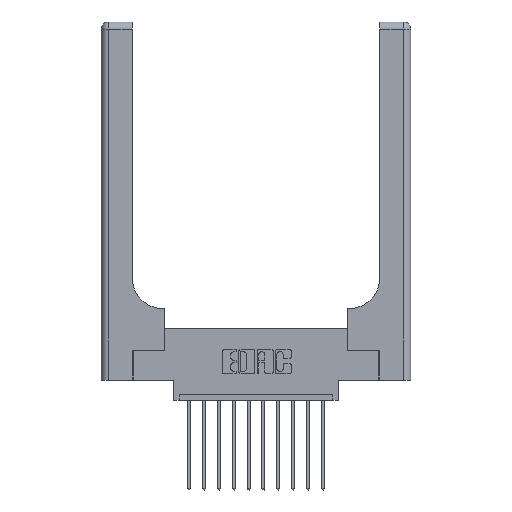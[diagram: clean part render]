
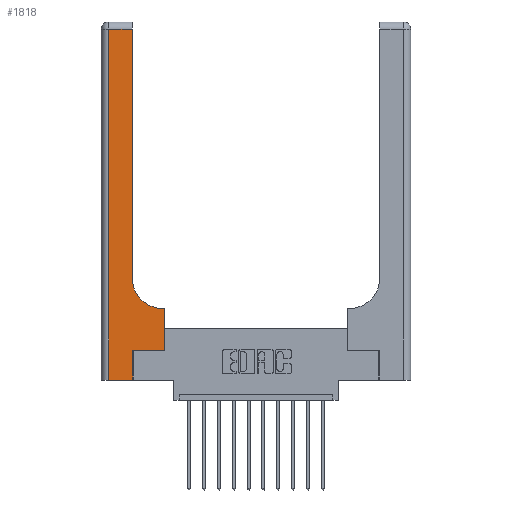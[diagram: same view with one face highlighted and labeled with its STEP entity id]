
A CAD part, top view. The second image highlights one B-rep face of the part: STEP entity #1818.
In plain terms, the highlighted planar face has unit normal (0, 0, 1).
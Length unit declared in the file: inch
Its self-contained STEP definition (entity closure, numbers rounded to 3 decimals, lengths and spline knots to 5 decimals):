
#231 = EDGE_CURVE ( 'NONE', #11655, #13411, #13240, .T. ) ;
#300 = DIRECTION ( 'NONE',  ( 1., 0., 0. ) ) ;
#375 = LINE ( 'NONE', #10136, #12994 ) ;
#502 = LINE ( 'NONE', #2709, #3537 ) ;
#524 = EDGE_LOOP ( 'NONE', ( #6672, #3732, #3920, #12503, #13921, #8784, #4140, #12211, #5558 ) ) ;
#971 = CARTESIAN_POINT ( 'NONE',  ( 0.06, 2.94, 0.37 ) ) ;
#1190 = LINE ( 'NONE', #6204, #11714 ) ;
#1419 = EDGE_CURVE ( 'NONE', #5916, #8251, #5658, .T. ) ;
#1541 = DIRECTION ( 'NONE',  ( 1., 0., 0. ) ) ;
#1778 = VECTOR ( 'NONE', #8860, 39.37008 ) ;
#1818 = ADVANCED_FACE ( 'NONE', ( #9662 ), #10863, .F. ) ;
#2227 = CARTESIAN_POINT ( 'NONE',  ( 0.51, 0.6, 0.37 ) ) ;
#2591 = CARTESIAN_POINT ( 'NONE',  ( 0.265, 0., 0.37 ) ) ;
#2709 = CARTESIAN_POINT ( 'NONE',  ( 0.26, 0.6, 0.37 ) ) ;
#3477 = EDGE_CURVE ( 'NONE', #13411, #10782, #11350, .T. ) ;
#3537 = VECTOR ( 'NONE', #4005, 39.37008 ) ;
#3730 = CARTESIAN_POINT ( 'NONE',  ( 0.528, 0.25, 0.37 ) ) ;
#3732 = ORIENTED_EDGE ( 'NONE', *, *, #231, .T. ) ;
#3757 = CARTESIAN_POINT ( 'NONE',  ( 0., 0., 0.37 ) ) ;
#3920 = ORIENTED_EDGE ( 'NONE', *, *, #3477, .T. ) ;
#4005 = DIRECTION ( 'NONE',  ( -1., 0., 0. ) ) ;
#4070 = EDGE_CURVE ( 'NONE', #8092, #7566, #1190, .T. ) ;
#4140 = ORIENTED_EDGE ( 'NONE', *, *, #1419, .T. ) ;
#4496 = EDGE_CURVE ( 'NONE', #8410, #8673, #9220, .T. ) ;
#4697 = CARTESIAN_POINT ( 'NONE',  ( 0., 3., 0.37 ) ) ;
#4716 = DIRECTION ( 'NONE',  ( 0., -1., 0. ) ) ;
#5558 = ORIENTED_EDGE ( 'NONE', *, *, #4496, .T. ) ;
#5658 = LINE ( 'NONE', #3730, #12937 ) ;
#5916 = VERTEX_POINT ( 'NONE', #9123 ) ;
#5938 = DIRECTION ( 'NONE',  ( 0., 0., -1. ) ) ;
#6204 = CARTESIAN_POINT ( 'NONE',  ( 0.265, 0., 0.37 ) ) ;
#6386 = CARTESIAN_POINT ( 'NONE',  ( 0.51, 0.85, 0.37 ) ) ;
#6549 = CARTESIAN_POINT ( 'NONE',  ( 0., 2.94, 0.37 ) ) ;
#6672 = ORIENTED_EDGE ( 'NONE', *, *, #13767, .T. ) ;
#7401 = DIRECTION ( 'NONE',  ( 0., 0., -1. ) ) ;
#7566 = VERTEX_POINT ( 'NONE', #10106 ) ;
#7866 = DIRECTION ( 'NONE',  ( 0., 1., 0. ) ) ;
#8092 = VERTEX_POINT ( 'NONE', #2591 ) ;
#8251 = VERTEX_POINT ( 'NONE', #9062 ) ;
#8410 = VERTEX_POINT ( 'NONE', #2227 ) ;
#8673 = VERTEX_POINT ( 'NONE', #8778 ) ;
#8778 = CARTESIAN_POINT ( 'NONE',  ( 0.26, 0.85, 0.37 ) ) ;
#8784 = ORIENTED_EDGE ( 'NONE', *, *, #11522, .T. ) ;
#8860 = DIRECTION ( 'NONE',  ( -1., 0., 0. ) ) ;
#9062 = CARTESIAN_POINT ( 'NONE',  ( 0.528, 0.6, 0.37 ) ) ;
#9123 = CARTESIAN_POINT ( 'NONE',  ( 0.528, 0.25, 0.37 ) ) ;
#9220 = CIRCLE ( 'NONE', #14341, 0.25 ) ;
#9400 = EDGE_CURVE ( 'NONE', #10782, #8092, #12499, .T. ) ;
#9460 = LINE ( 'NONE', #12733, #11780 ) ;
#9534 = CARTESIAN_POINT ( 'NONE',  ( 0.06, 0., 0.37 ) ) ;
#9662 = FACE_OUTER_BOUND ( 'NONE', #524, .T. ) ;
#9949 = DIRECTION ( 'NONE',  ( 0., 1., 0. ) ) ;
#10106 = CARTESIAN_POINT ( 'NONE',  ( 0.265, 0.25, 0.37 ) ) ;
#10136 = CARTESIAN_POINT ( 'NONE',  ( 0.265, 0.25, 0.37 ) ) ;
#10161 = DIRECTION ( 'NONE',  ( 0., 1., 0. ) ) ;
#10782 = VERTEX_POINT ( 'NONE', #9534 ) ;
#10863 = PLANE ( 'NONE',  #13184 ) ;
#11350 = LINE ( 'NONE', #15712, #14219 ) ;
#11522 = EDGE_CURVE ( 'NONE', #7566, #5916, #375, .T. ) ;
#11637 = CARTESIAN_POINT ( 'NONE',  ( 0.26, 2.94, 0.37 ) ) ;
#11655 = VERTEX_POINT ( 'NONE', #11637 ) ;
#11714 = VECTOR ( 'NONE', #9949, 39.37008 ) ;
#11726 = VECTOR ( 'NONE', #14881, 39.37008 ) ;
#11780 = VECTOR ( 'NONE', #10161, 39.37008 ) ;
#12211 = ORIENTED_EDGE ( 'NONE', *, *, #13562, .T. ) ;
#12499 = LINE ( 'NONE', #3757, #11726 ) ;
#12503 = ORIENTED_EDGE ( 'NONE', *, *, #9400, .T. ) ;
#12733 = CARTESIAN_POINT ( 'NONE',  ( 0.26, 3., 0.37 ) ) ;
#12937 = VECTOR ( 'NONE', #7866, 39.37008 ) ;
#12994 = VECTOR ( 'NONE', #300, 39.37008 ) ;
#13184 = AXIS2_PLACEMENT_3D ( 'NONE', #4697, #5938, #15743 ) ;
#13240 = LINE ( 'NONE', #6549, #1778 ) ;
#13411 = VERTEX_POINT ( 'NONE', #971 ) ;
#13562 = EDGE_CURVE ( 'NONE', #8251, #8410, #502, .T. ) ;
#13767 = EDGE_CURVE ( 'NONE', #8673, #11655, #9460, .T. ) ;
#13921 = ORIENTED_EDGE ( 'NONE', *, *, #4070, .T. ) ;
#14219 = VECTOR ( 'NONE', #4716, 39.37008 ) ;
#14341 = AXIS2_PLACEMENT_3D ( 'NONE', #6386, #7401, #1541 ) ;
#14881 = DIRECTION ( 'NONE',  ( 1., 0., 0. ) ) ;
#15712 = CARTESIAN_POINT ( 'NONE',  ( 0.06, 3., 0.37 ) ) ;
#15743 = DIRECTION ( 'NONE',  ( -1., 0., 0. ) ) ;
